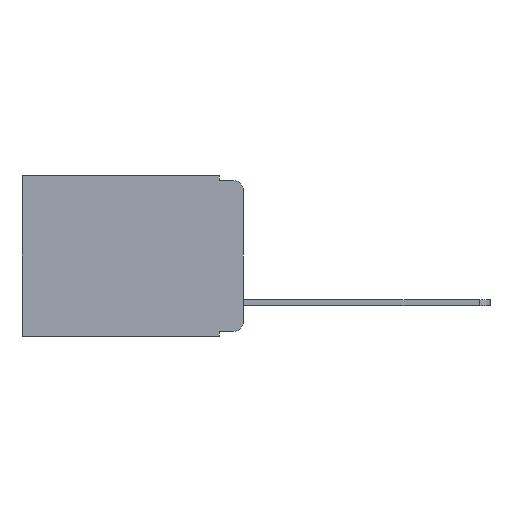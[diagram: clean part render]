
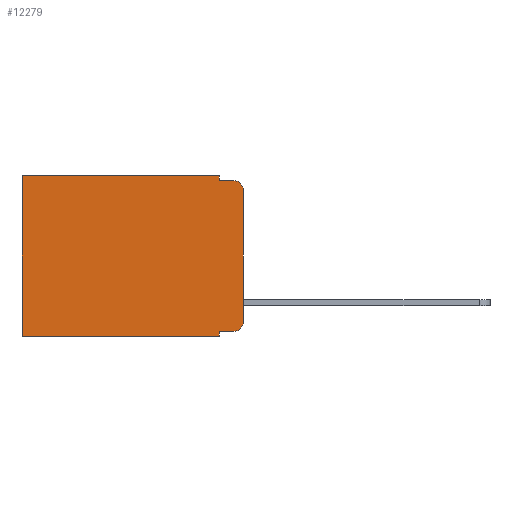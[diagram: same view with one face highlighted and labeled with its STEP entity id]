
A CAD part, left-side view. The second image highlights one B-rep face of the part: STEP entity #12279.
In plain terms, the highlighted planar face has unit normal (-1, 0, 0).
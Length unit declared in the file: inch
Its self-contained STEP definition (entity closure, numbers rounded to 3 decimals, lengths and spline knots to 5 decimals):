
#105 = DIRECTION ( 'NONE',  ( 0., 0., -1. ) ) ;
#231 = CARTESIAN_POINT ( 'NONE',  ( 0.298, 0.02, -0.333 ) ) ;
#273 = LINE ( 'NONE', #10049, #11694 ) ;
#292 = VERTEX_POINT ( 'NONE', #12114 ) ;
#418 = ORIENTED_EDGE ( 'NONE', *, *, #11080, .F. ) ;
#502 = EDGE_CURVE ( 'NONE', #3468, #12786, #4972, .T. ) ;
#531 = EDGE_LOOP ( 'NONE', ( #418, #9288, #1134, #9992, #7350, #10698, #5173, #13844, #8411, #8762 ) ) ;
#616 = LINE ( 'NONE', #11546, #9107 ) ;
#699 = CIRCLE ( 'NONE', #9366, 0.02 ) ;
#902 = CARTESIAN_POINT ( 'NONE',  ( 0.298, 0.051, 0. ) ) ;
#1134 = ORIENTED_EDGE ( 'NONE', *, *, #8203, .F. ) ;
#1180 = LINE ( 'NONE', #11767, #12538 ) ;
#1724 = CARTESIAN_POINT ( 'NONE',  ( 0.298, 0.02, -0.01 ) ) ;
#2011 = VECTOR ( 'NONE', #3016, 39.37008 ) ;
#2275 = LINE ( 'NONE', #4761, #7766 ) ;
#2470 = LINE ( 'NONE', #4845, #7978 ) ;
#2574 = VERTEX_POINT ( 'NONE', #13427 ) ;
#2602 = CARTESIAN_POINT ( 'NONE',  ( 0.298, 0.051, -0.343 ) ) ;
#3016 = DIRECTION ( 'NONE',  ( 0., -1., 0. ) ) ;
#3018 = VERTEX_POINT ( 'NONE', #5800 ) ;
#3085 = VERTEX_POINT ( 'NONE', #2602 ) ;
#3218 = CARTESIAN_POINT ( 'NONE',  ( 0.298, 0.473, 0. ) ) ;
#3238 = VERTEX_POINT ( 'NONE', #8385 ) ;
#3468 = VERTEX_POINT ( 'NONE', #4454 ) ;
#3847 = DIRECTION ( 'NONE',  ( 0., 0., -1. ) ) ;
#3911 = EDGE_CURVE ( 'NONE', #4566, #10009, #1180, .T. ) ;
#4454 = CARTESIAN_POINT ( 'NONE',  ( 0.298, 0.051, -0.333 ) ) ;
#4566 = VERTEX_POINT ( 'NONE', #902 ) ;
#4688 = CIRCLE ( 'NONE', #9529, 0.02 ) ;
#4721 = DIRECTION ( 'NONE',  ( -1., 0., 0. ) ) ;
#4761 = CARTESIAN_POINT ( 'NONE',  ( 0.298, 0.051, 0. ) ) ;
#4770 = VECTOR ( 'NONE', #9836, 39.37008 ) ;
#4845 = CARTESIAN_POINT ( 'NONE',  ( 0.298, 0., 0. ) ) ;
#4972 = LINE ( 'NONE', #8643, #2011 ) ;
#5173 = ORIENTED_EDGE ( 'NONE', *, *, #7266, .F. ) ;
#5231 = VERTEX_POINT ( 'NONE', #1724 ) ;
#5615 = LINE ( 'NONE', #7857, #8879 ) ;
#5715 = CARTESIAN_POINT ( 'NONE',  ( 0.298, 0.02, -0.313 ) ) ;
#5800 = CARTESIAN_POINT ( 'NONE',  ( 0.298, 0., -0.03 ) ) ;
#5930 = DIRECTION ( 'NONE',  ( 0., 0., -1. ) ) ;
#6708 = EDGE_CURVE ( 'NONE', #3018, #5231, #4688, .T. ) ;
#6716 = DIRECTION ( 'NONE',  ( 0., 1., 0. ) ) ;
#6776 = DIRECTION ( 'NONE',  ( 0., 0., -1. ) ) ;
#7266 = EDGE_CURVE ( 'NONE', #3085, #292, #273, .T. ) ;
#7273 = AXIS2_PLACEMENT_3D ( 'NONE', #9333, #10468, #3847 ) ;
#7296 = LINE ( 'NONE', #3218, #4770 ) ;
#7350 = ORIENTED_EDGE ( 'NONE', *, *, #3911, .T. ) ;
#7766 = VECTOR ( 'NONE', #10310, 39.37008 ) ;
#7857 = CARTESIAN_POINT ( 'NONE',  ( 0.298, 0.051, 0. ) ) ;
#7978 = VECTOR ( 'NONE', #5930, 39.37008 ) ;
#8199 = PLANE ( 'NONE',  #7273 ) ;
#8203 = EDGE_CURVE ( 'NONE', #3238, #5231, #616, .T. ) ;
#8385 = CARTESIAN_POINT ( 'NONE',  ( 0.298, 0.051, -0.01 ) ) ;
#8411 = ORIENTED_EDGE ( 'NONE', *, *, #502, .T. ) ;
#8643 = CARTESIAN_POINT ( 'NONE',  ( 0.298, 0.051, -0.333 ) ) ;
#8762 = ORIENTED_EDGE ( 'NONE', *, *, #13936, .T. ) ;
#8879 = VECTOR ( 'NONE', #105, 39.37008 ) ;
#9107 = VECTOR ( 'NONE', #9400, 39.37008 ) ;
#9288 = ORIENTED_EDGE ( 'NONE', *, *, #6708, .T. ) ;
#9333 = CARTESIAN_POINT ( 'NONE',  ( 0.298, 0., 0. ) ) ;
#9366 = AXIS2_PLACEMENT_3D ( 'NONE', #5715, #13326, #6776 ) ;
#9400 = DIRECTION ( 'NONE',  ( 0., -1., 0. ) ) ;
#9529 = AXIS2_PLACEMENT_3D ( 'NONE', #11303, #4721, #12344 ) ;
#9836 = DIRECTION ( 'NONE',  ( 0., 0., -1. ) ) ;
#9992 = ORIENTED_EDGE ( 'NONE', *, *, #10472, .F. ) ;
#10009 = VERTEX_POINT ( 'NONE', #12605 ) ;
#10049 = CARTESIAN_POINT ( 'NONE',  ( 0.298, 0., -0.343 ) ) ;
#10310 = DIRECTION ( 'NONE',  ( 0., 0., -1. ) ) ;
#10468 = DIRECTION ( 'NONE',  ( 1., 0., 0. ) ) ;
#10472 = EDGE_CURVE ( 'NONE', #4566, #3238, #5615, .T. ) ;
#10698 = ORIENTED_EDGE ( 'NONE', *, *, #12588, .T. ) ;
#10720 = DIRECTION ( 'NONE',  ( 0., 1., 0. ) ) ;
#11080 = EDGE_CURVE ( 'NONE', #3018, #2574, #2470, .T. ) ;
#11149 = FACE_OUTER_BOUND ( 'NONE', #531, .T. ) ;
#11303 = CARTESIAN_POINT ( 'NONE',  ( 0.298, 0.02, -0.03 ) ) ;
#11546 = CARTESIAN_POINT ( 'NONE',  ( 0.298, 0.051, -0.01 ) ) ;
#11694 = VECTOR ( 'NONE', #6716, 39.37008 ) ;
#11767 = CARTESIAN_POINT ( 'NONE',  ( 0.298, 0., 0. ) ) ;
#12114 = CARTESIAN_POINT ( 'NONE',  ( 0.298, 0.473, -0.343 ) ) ;
#12279 = ADVANCED_FACE ( 'NONE', ( #11149 ), #8199, .F. ) ;
#12344 = DIRECTION ( 'NONE',  ( 0., 0., -1. ) ) ;
#12538 = VECTOR ( 'NONE', #10720, 39.37008 ) ;
#12588 = EDGE_CURVE ( 'NONE', #10009, #292, #7296, .T. ) ;
#12605 = CARTESIAN_POINT ( 'NONE',  ( 0.298, 0.473, 0. ) ) ;
#12786 = VERTEX_POINT ( 'NONE', #231 ) ;
#13326 = DIRECTION ( 'NONE',  ( -1., 0., 0. ) ) ;
#13427 = CARTESIAN_POINT ( 'NONE',  ( 0.298, 0., -0.313 ) ) ;
#13844 = ORIENTED_EDGE ( 'NONE', *, *, #14043, .F. ) ;
#13936 = EDGE_CURVE ( 'NONE', #12786, #2574, #699, .T. ) ;
#14043 = EDGE_CURVE ( 'NONE', #3468, #3085, #2275, .T. ) ;
